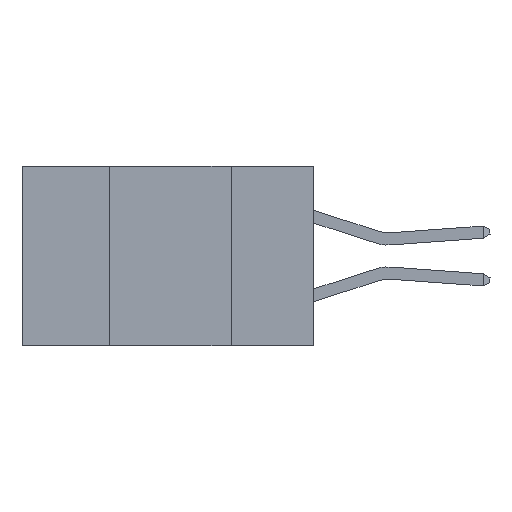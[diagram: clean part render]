
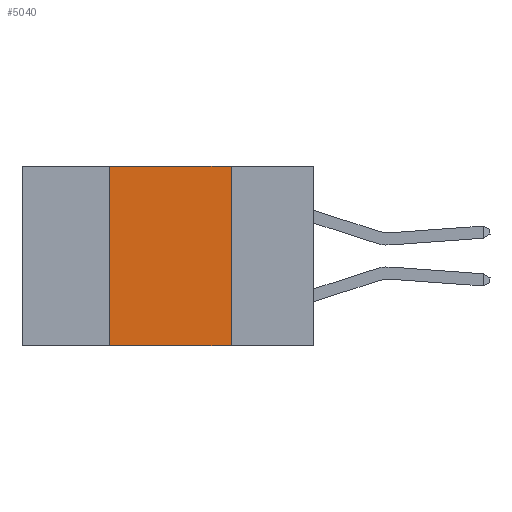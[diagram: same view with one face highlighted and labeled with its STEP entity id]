
A CAD part, left-side view. The second image highlights one B-rep face of the part: STEP entity #5040.
In plain terms, the highlighted planar face has unit normal (-1, 0, 0).
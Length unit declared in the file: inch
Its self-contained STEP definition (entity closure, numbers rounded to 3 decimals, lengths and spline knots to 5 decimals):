
#304 = LINE ( 'NONE', #4500, #5800 ) ;
#395 = VECTOR ( 'NONE', #14765, 39.37008 ) ;
#664 = VECTOR ( 'NONE', #4376, 39.37008 ) ;
#1442 = ORIENTED_EDGE ( 'NONE', *, *, #7623, .F. ) ;
#1632 = ORIENTED_EDGE ( 'NONE', *, *, #17634, .F. ) ;
#1988 = ORIENTED_EDGE ( 'NONE', *, *, #2936, .F. ) ;
#2045 = LINE ( 'NONE', #18829, #12446 ) ;
#2334 = CARTESIAN_POINT ( 'NONE',  ( 0., 0.6, 0. ) ) ;
#2936 = EDGE_CURVE ( 'NONE', #18250, #11283, #16894, .T. ) ;
#3127 = VERTEX_POINT ( 'NONE', #5020 ) ;
#4376 = DIRECTION ( 'NONE',  ( 0., -1., 0. ) ) ;
#4500 = CARTESIAN_POINT ( 'NONE',  ( 0., 0.42, 0. ) ) ;
#4916 = FACE_OUTER_BOUND ( 'NONE', #9677, .T. ) ;
#5020 = CARTESIAN_POINT ( 'NONE',  ( 0., 0.42, -0.37 ) ) ;
#5040 = ADVANCED_FACE ( 'NONE', ( #4916 ), #6794, .F. ) ;
#5800 = VECTOR ( 'NONE', #21069, 39.37008 ) ;
#6794 = PLANE ( 'NONE',  #20854 ) ;
#7623 = EDGE_CURVE ( 'NONE', #3127, #19629, #304, .T. ) ;
#8886 = DIRECTION ( 'NONE',  ( 0., 0., -1. ) ) ;
#9677 = EDGE_LOOP ( 'NONE', ( #1988, #1632, #1442, #11349 ) ) ;
#10543 = CARTESIAN_POINT ( 'NONE',  ( 0., 0.17, -0.37 ) ) ;
#11283 = VERTEX_POINT ( 'NONE', #10543 ) ;
#11349 = ORIENTED_EDGE ( 'NONE', *, *, #12042, .T. ) ;
#12042 = EDGE_CURVE ( 'NONE', #3127, #11283, #2045, .T. ) ;
#12344 = LINE ( 'NONE', #2334, #664 ) ;
#12446 = VECTOR ( 'NONE', #22909, 39.37008 ) ;
#13742 = CARTESIAN_POINT ( 'NONE',  ( 0., 0.42, 0. ) ) ;
#14765 = DIRECTION ( 'NONE',  ( 0., 0., -1. ) ) ;
#16894 = LINE ( 'NONE', #20796, #395 ) ;
#17036 = CARTESIAN_POINT ( 'NONE',  ( 0., 0.17, 0. ) ) ;
#17634 = EDGE_CURVE ( 'NONE', #19629, #18250, #12344, .T. ) ;
#18250 = VERTEX_POINT ( 'NONE', #17036 ) ;
#18829 = CARTESIAN_POINT ( 'NONE',  ( 0., 0.6, -0.37 ) ) ;
#19629 = VERTEX_POINT ( 'NONE', #13742 ) ;
#20796 = CARTESIAN_POINT ( 'NONE',  ( 0., 0.17, 0. ) ) ;
#20854 = AXIS2_PLACEMENT_3D ( 'NONE', #25151, #21149, #8886 ) ;
#21069 = DIRECTION ( 'NONE',  ( 0., 0., 1. ) ) ;
#21149 = DIRECTION ( 'NONE',  ( 1., 0., 0. ) ) ;
#22909 = DIRECTION ( 'NONE',  ( 0., -1., 0. ) ) ;
#25151 = CARTESIAN_POINT ( 'NONE',  ( 0., 0.6, 0. ) ) ;
